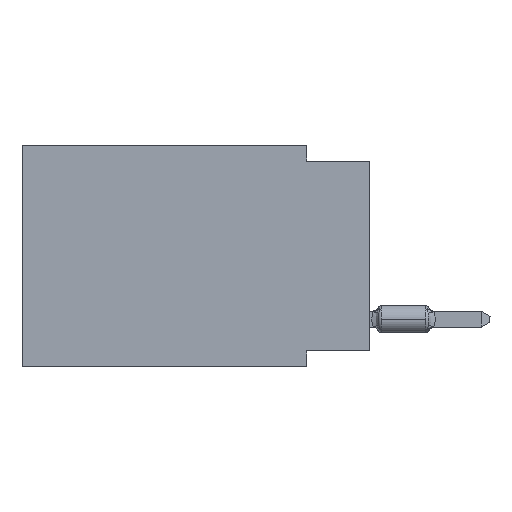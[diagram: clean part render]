
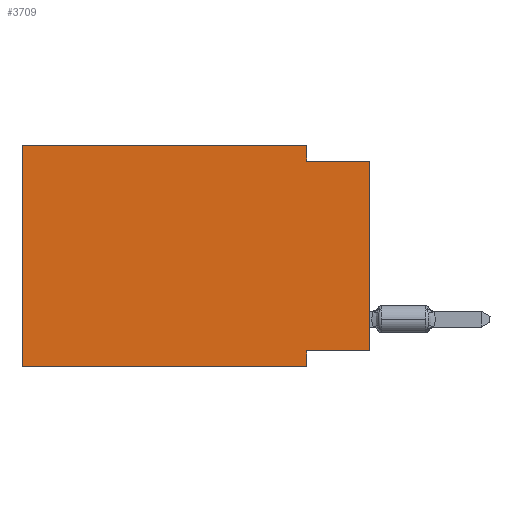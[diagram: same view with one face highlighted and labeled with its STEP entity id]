
A CAD part, left-side view. The second image highlights one B-rep face of the part: STEP entity #3709.
In plain terms, the highlighted planar face has unit normal (-1, 0, 0).
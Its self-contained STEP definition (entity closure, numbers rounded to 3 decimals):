
#260 = VERTEX_POINT ( 'NONE', #7870 ) ;
#1362 = VECTOR ( 'NONE', #1706, 1000. ) ;
#1706 = DIRECTION ( 'NONE',  ( 0., 0., 1. ) ) ;
#2013 = LINE ( 'NONE', #32609, #30263 ) ;
#2453 = CARTESIAN_POINT ( 'NONE',  ( 0., 2.54, -8.255 ) ) ;
#3516 = CARTESIAN_POINT ( 'NONE',  ( 0., 13.97, -8.89 ) ) ;
#3709 = ADVANCED_FACE ( 'NONE', ( #28258 ), #30816, .F. ) ;
#5004 = LINE ( 'NONE', #8118, #11286 ) ;
#5417 = DIRECTION ( 'NONE',  ( 0., 0., -1. ) ) ;
#5872 = CARTESIAN_POINT ( 'NONE',  ( 0., 13.97, 0. ) ) ;
#6393 = VECTOR ( 'NONE', #22224, 1000. ) ;
#6421 = DIRECTION ( 'NONE',  ( 1., 0., 0. ) ) ;
#6572 = EDGE_CURVE ( 'NONE', #11769, #22459, #8765, .T. ) ;
#7042 = ORIENTED_EDGE ( 'NONE', *, *, #19249, .T. ) ;
#7691 = EDGE_CURVE ( 'NONE', #22459, #27969, #2013, .T. ) ;
#7870 = CARTESIAN_POINT ( 'NONE',  ( 0., 0., -8.255 ) ) ;
#8118 = CARTESIAN_POINT ( 'NONE',  ( 0., 0., -8.255 ) ) ;
#8589 = ORIENTED_EDGE ( 'NONE', *, *, #26947, .F. ) ;
#8765 = LINE ( 'NONE', #13684, #6393 ) ;
#10199 = EDGE_CURVE ( 'NONE', #30569, #11813, #27928, .T. ) ;
#10981 = CARTESIAN_POINT ( 'NONE',  ( 0., 13.97, 0. ) ) ;
#11286 = VECTOR ( 'NONE', #16119, 1000. ) ;
#11769 = VERTEX_POINT ( 'NONE', #24069 ) ;
#11813 = VERTEX_POINT ( 'NONE', #10981 ) ;
#12472 = LINE ( 'NONE', #20649, #18873 ) ;
#12843 = CARTESIAN_POINT ( 'NONE',  ( 0., 2.54, -8.89 ) ) ;
#13684 = CARTESIAN_POINT ( 'NONE',  ( 0., 2.54, 0. ) ) ;
#15211 = VECTOR ( 'NONE', #5417, 1000. ) ;
#15706 = ORIENTED_EDGE ( 'NONE', *, *, #29990, .F. ) ;
#15960 = ORIENTED_EDGE ( 'NONE', *, *, #7691, .F. ) ;
#16119 = DIRECTION ( 'NONE',  ( 0., 1., 0. ) ) ;
#16809 = LINE ( 'NONE', #3516, #18902 ) ;
#17006 = DIRECTION ( 'NONE',  ( 0., 0., 1. ) ) ;
#17784 = ORIENTED_EDGE ( 'NONE', *, *, #25537, .F. ) ;
#18729 = CARTESIAN_POINT ( 'NONE',  ( 0., 0., -0.635 ) ) ;
#18873 = VECTOR ( 'NONE', #26652, 1000. ) ;
#18902 = VECTOR ( 'NONE', #27911, 1000. ) ;
#19249 = EDGE_CURVE ( 'NONE', #260, #27969, #20481, .T. ) ;
#19288 = VERTEX_POINT ( 'NONE', #12843 ) ;
#20481 = LINE ( 'NONE', #34850, #1362 ) ;
#20649 = CARTESIAN_POINT ( 'NONE',  ( 0., 13.97, 0. ) ) ;
#22224 = DIRECTION ( 'NONE',  ( 0., 0., -1. ) ) ;
#22459 = VERTEX_POINT ( 'NONE', #34268 ) ;
#24069 = CARTESIAN_POINT ( 'NONE',  ( 0., 2.54, 0. ) ) ;
#25533 = DIRECTION ( 'NONE',  ( 0., 0., -1. ) ) ;
#25537 = EDGE_CURVE ( 'NONE', #260, #28753, #5004, .T. ) ;
#26652 = DIRECTION ( 'NONE',  ( 0., -1., 0. ) ) ;
#26947 = EDGE_CURVE ( 'NONE', #11813, #11769, #12472, .T. ) ;
#27184 = EDGE_CURVE ( 'NONE', #30569, #19288, #16809, .T. ) ;
#27911 = DIRECTION ( 'NONE',  ( 0., -1., 0. ) ) ;
#27928 = LINE ( 'NONE', #35939, #30156 ) ;
#27969 = VERTEX_POINT ( 'NONE', #18729 ) ;
#28258 = FACE_OUTER_BOUND ( 'NONE', #33565, .T. ) ;
#28753 = VERTEX_POINT ( 'NONE', #2453 ) ;
#29879 = DIRECTION ( 'NONE',  ( 0., -1., 0. ) ) ;
#29990 = EDGE_CURVE ( 'NONE', #28753, #19288, #33446, .T. ) ;
#30156 = VECTOR ( 'NONE', #17006, 1000. ) ;
#30185 = CARTESIAN_POINT ( 'NONE',  ( 0., 2.54, -8.89 ) ) ;
#30263 = VECTOR ( 'NONE', #29879, 1000. ) ;
#30569 = VERTEX_POINT ( 'NONE', #31888 ) ;
#30816 = PLANE ( 'NONE',  #33546 ) ;
#31317 = ORIENTED_EDGE ( 'NONE', *, *, #6572, .F. ) ;
#31888 = CARTESIAN_POINT ( 'NONE',  ( 0., 13.97, -8.89 ) ) ;
#31934 = ORIENTED_EDGE ( 'NONE', *, *, #10199, .F. ) ;
#32609 = CARTESIAN_POINT ( 'NONE',  ( 0., 0., -0.635 ) ) ;
#33345 = ORIENTED_EDGE ( 'NONE', *, *, #27184, .T. ) ;
#33446 = LINE ( 'NONE', #30185, #15211 ) ;
#33546 = AXIS2_PLACEMENT_3D ( 'NONE', #5872, #6421, #25533 ) ;
#33565 = EDGE_LOOP ( 'NONE', ( #7042, #15960, #31317, #8589, #31934, #33345, #15706, #17784 ) ) ;
#34268 = CARTESIAN_POINT ( 'NONE',  ( 0., 2.54, -0.635 ) ) ;
#34850 = CARTESIAN_POINT ( 'NONE',  ( 0., 0., 0. ) ) ;
#35939 = CARTESIAN_POINT ( 'NONE',  ( 0., 13.97, 0. ) ) ;
